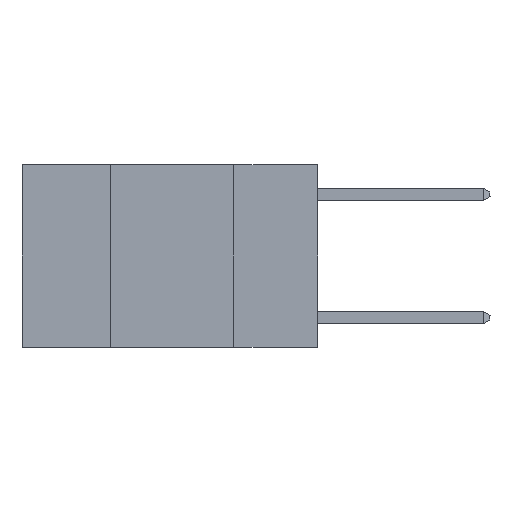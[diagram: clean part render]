
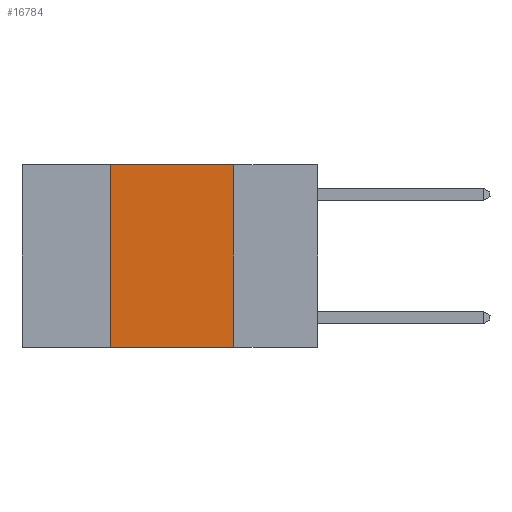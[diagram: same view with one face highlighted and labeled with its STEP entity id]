
A CAD part, left-side view. The second image highlights one B-rep face of the part: STEP entity #16784.
In plain terms, the highlighted planar face has unit normal (-1, 0, 0).
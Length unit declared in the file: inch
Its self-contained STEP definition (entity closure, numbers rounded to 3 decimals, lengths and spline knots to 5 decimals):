
#118 = CARTESIAN_POINT ( 'NONE',  ( 0., 0.6, 0. ) ) ;
#472 = CARTESIAN_POINT ( 'NONE',  ( 0., 0.42, 0. ) ) ;
#623 = ORIENTED_EDGE ( 'NONE', *, *, #6293, .F. ) ;
#3112 = VECTOR ( 'NONE', #8446, 39.37008 ) ;
#5053 = VERTEX_POINT ( 'NONE', #472 ) ;
#5344 = FACE_OUTER_BOUND ( 'NONE', #13611, .T. ) ;
#5748 = EDGE_CURVE ( 'NONE', #21616, #5053, #22698, .T. ) ;
#6293 = EDGE_CURVE ( 'NONE', #5053, #21956, #16196, .T. ) ;
#8016 = VERTEX_POINT ( 'NONE', #20938 ) ;
#8162 = VECTOR ( 'NONE', #13047, 39.37008 ) ;
#8446 = DIRECTION ( 'NONE',  ( 0., 0., -1. ) ) ;
#8887 = VECTOR ( 'NONE', #12482, 39.37008 ) ;
#8915 = AXIS2_PLACEMENT_3D ( 'NONE', #118, #10434, #17509 ) ;
#10089 = VECTOR ( 'NONE', #14957, 39.37008 ) ;
#10434 = DIRECTION ( 'NONE',  ( 1., 0., 0. ) ) ;
#10835 = EDGE_CURVE ( 'NONE', #21956, #8016, #13554, .T. ) ;
#11199 = ORIENTED_EDGE ( 'NONE', *, *, #5748, .F. ) ;
#11582 = CARTESIAN_POINT ( 'NONE',  ( 0., 0.17, 0. ) ) ;
#12482 = DIRECTION ( 'NONE',  ( 0., 0., 1. ) ) ;
#12810 = CARTESIAN_POINT ( 'NONE',  ( 0., 0.6, 0. ) ) ;
#13047 = DIRECTION ( 'NONE',  ( 0., -1., 0. ) ) ;
#13554 = LINE ( 'NONE', #11582, #3112 ) ;
#13611 = EDGE_LOOP ( 'NONE', ( #13770, #623, #11199, #19781 ) ) ;
#13770 = ORIENTED_EDGE ( 'NONE', *, *, #10835, .F. ) ;
#14136 = PLANE ( 'NONE',  #8915 ) ;
#14957 = DIRECTION ( 'NONE',  ( 0., -1., 0. ) ) ;
#16196 = LINE ( 'NONE', #12810, #8162 ) ;
#16784 = ADVANCED_FACE ( 'NONE', ( #5344 ), #14136, .F. ) ;
#17349 = CARTESIAN_POINT ( 'NONE',  ( 0., 0.42, 0. ) ) ;
#17509 = DIRECTION ( 'NONE',  ( 0., 0., -1. ) ) ;
#19289 = EDGE_CURVE ( 'NONE', #21616, #8016, #20194, .T. ) ;
#19307 = CARTESIAN_POINT ( 'NONE',  ( 0., 0.17, 0. ) ) ;
#19781 = ORIENTED_EDGE ( 'NONE', *, *, #19289, .T. ) ;
#20194 = LINE ( 'NONE', #21935, #10089 ) ;
#20258 = CARTESIAN_POINT ( 'NONE',  ( 0., 0.42, -0.37 ) ) ;
#20938 = CARTESIAN_POINT ( 'NONE',  ( 0., 0.17, -0.37 ) ) ;
#21616 = VERTEX_POINT ( 'NONE', #20258 ) ;
#21935 = CARTESIAN_POINT ( 'NONE',  ( 0., 0.6, -0.37 ) ) ;
#21956 = VERTEX_POINT ( 'NONE', #19307 ) ;
#22698 = LINE ( 'NONE', #17349, #8887 ) ;
